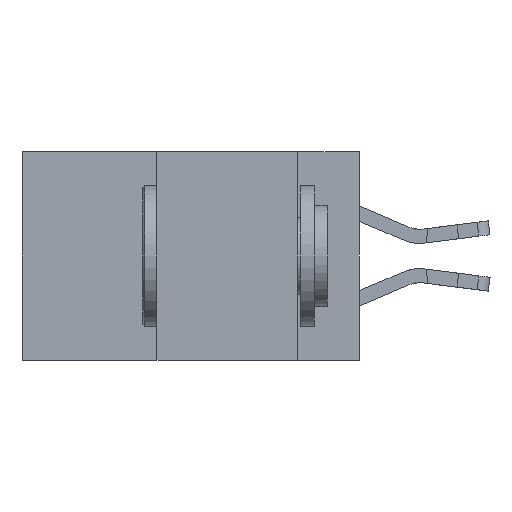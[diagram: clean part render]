
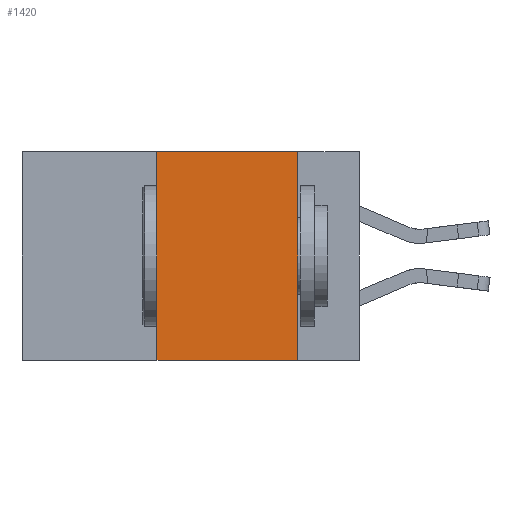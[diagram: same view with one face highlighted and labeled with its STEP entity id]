
A CAD part, left-side view. The second image highlights one B-rep face of the part: STEP entity #1420.
In plain terms, the highlighted planar face has unit normal (-1, 0, 0).
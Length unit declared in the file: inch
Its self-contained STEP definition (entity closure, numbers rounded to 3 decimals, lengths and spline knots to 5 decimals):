
#656 = CARTESIAN_POINT ( 'NONE',  ( 0., 0.36, 0. ) ) ;
#707 = ORIENTED_EDGE ( 'NONE', *, *, #15010, .F. ) ;
#779 = VERTEX_POINT ( 'NONE', #7276 ) ;
#1331 = EDGE_CURVE ( 'NONE', #779, #5071, #16747, .T. ) ;
#1420 = ADVANCED_FACE ( 'NONE', ( #19009 ), #12982, .F. ) ;
#1949 = ORIENTED_EDGE ( 'NONE', *, *, #1331, .F. ) ;
#2004 = VECTOR ( 'NONE', #10567, 39.37008 ) ;
#3420 = VECTOR ( 'NONE', #8007, 39.37008 ) ;
#3587 = LINE ( 'NONE', #9897, #20687 ) ;
#5071 = VERTEX_POINT ( 'NONE', #13663 ) ;
#6728 = EDGE_CURVE ( 'NONE', #7465, #17446, #3587, .T. ) ;
#7219 = EDGE_CURVE ( 'NONE', #7465, #779, #21177, .T. ) ;
#7276 = CARTESIAN_POINT ( 'NONE',  ( 0., 0.36, 0. ) ) ;
#7465 = VERTEX_POINT ( 'NONE', #7794 ) ;
#7794 = CARTESIAN_POINT ( 'NONE',  ( 0., 0.36, -0.37 ) ) ;
#8007 = DIRECTION ( 'NONE',  ( 0., -1., 0. ) ) ;
#9052 = CARTESIAN_POINT ( 'NONE',  ( 0., 0.11, 0. ) ) ;
#9897 = CARTESIAN_POINT ( 'NONE',  ( 0., 0.6, -0.37 ) ) ;
#10567 = DIRECTION ( 'NONE',  ( 0., 0., -1. ) ) ;
#10847 = AXIS2_PLACEMENT_3D ( 'NONE', #13047, #13445, #13102 ) ;
#11946 = ORIENTED_EDGE ( 'NONE', *, *, #7219, .F. ) ;
#12982 = PLANE ( 'NONE',  #10847 ) ;
#13047 = CARTESIAN_POINT ( 'NONE',  ( 0., 0.6, 0. ) ) ;
#13102 = DIRECTION ( 'NONE',  ( 0., 0., -1. ) ) ;
#13445 = DIRECTION ( 'NONE',  ( 1., 0., 0. ) ) ;
#13546 = CARTESIAN_POINT ( 'NONE',  ( 0., 0.6, 0. ) ) ;
#13663 = CARTESIAN_POINT ( 'NONE',  ( 0., 0.11, 0. ) ) ;
#14033 = CARTESIAN_POINT ( 'NONE',  ( 0., 0.11, -0.37 ) ) ;
#14215 = DIRECTION ( 'NONE',  ( 0., 0., 1. ) ) ;
#15010 = EDGE_CURVE ( 'NONE', #5071, #17446, #20240, .T. ) ;
#15275 = EDGE_LOOP ( 'NONE', ( #707, #1949, #11946, #20936 ) ) ;
#16353 = VECTOR ( 'NONE', #14215, 39.37008 ) ;
#16747 = LINE ( 'NONE', #13546, #3420 ) ;
#17446 = VERTEX_POINT ( 'NONE', #14033 ) ;
#18088 = DIRECTION ( 'NONE',  ( 0., -1., 0. ) ) ;
#19009 = FACE_OUTER_BOUND ( 'NONE', #15275, .T. ) ;
#20240 = LINE ( 'NONE', #9052, #2004 ) ;
#20687 = VECTOR ( 'NONE', #18088, 39.37008 ) ;
#20936 = ORIENTED_EDGE ( 'NONE', *, *, #6728, .T. ) ;
#21177 = LINE ( 'NONE', #656, #16353 ) ;
